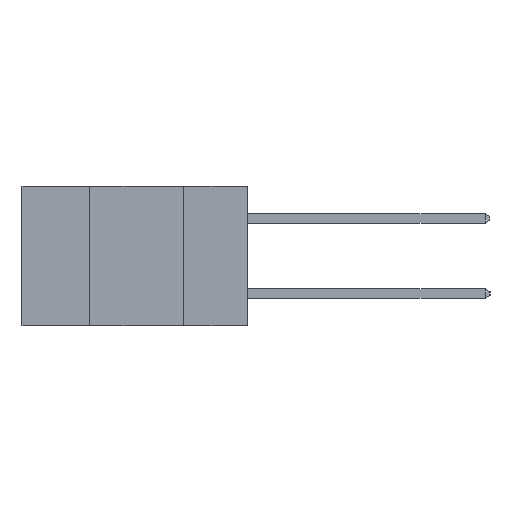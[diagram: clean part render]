
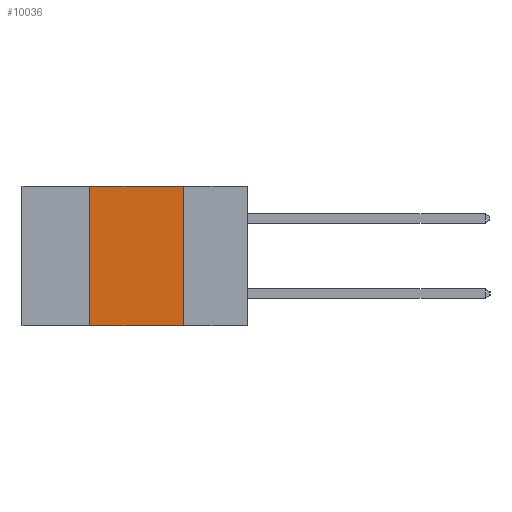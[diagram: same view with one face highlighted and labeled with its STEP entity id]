
A CAD part, left-side view. The second image highlights one B-rep face of the part: STEP entity #10036.
In plain terms, the highlighted planar face has unit normal (-1, 0, 0).
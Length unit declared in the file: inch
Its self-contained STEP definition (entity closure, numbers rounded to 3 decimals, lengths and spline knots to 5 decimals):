
#439 = CARTESIAN_POINT ( 'NONE',  ( 0., 0.42, 0. ) ) ;
#570 = VECTOR ( 'NONE', #14172, 39.37008 ) ;
#571 = DIRECTION ( 'NONE',  ( 0., 0., 1. ) ) ;
#798 = ORIENTED_EDGE ( 'NONE', *, *, #13704, .T. ) ;
#988 = ORIENTED_EDGE ( 'NONE', *, *, #10927, .F. ) ;
#1127 = CARTESIAN_POINT ( 'NONE',  ( 0., 0.6, -0.37 ) ) ;
#1369 = VERTEX_POINT ( 'NONE', #439 ) ;
#2080 = ORIENTED_EDGE ( 'NONE', *, *, #7025, .F. ) ;
#2158 = CARTESIAN_POINT ( 'NONE',  ( 0., 0.42, -0.37 ) ) ;
#2432 = ORIENTED_EDGE ( 'NONE', *, *, #4763, .F. ) ;
#2491 = VERTEX_POINT ( 'NONE', #6785 ) ;
#3468 = DIRECTION ( 'NONE',  ( 0., 0., -1. ) ) ;
#3516 = CARTESIAN_POINT ( 'NONE',  ( 0., 0.17, -0.37 ) ) ;
#4007 = EDGE_LOOP ( 'NONE', ( #2432, #988, #2080, #798 ) ) ;
#4614 = AXIS2_PLACEMENT_3D ( 'NONE', #9665, #9629, #12897 ) ;
#4763 = EDGE_CURVE ( 'NONE', #11511, #11398, #11446, .T. ) ;
#6702 = VECTOR ( 'NONE', #9638, 39.37008 ) ;
#6785 = CARTESIAN_POINT ( 'NONE',  ( 0., 0.42, -0.37 ) ) ;
#7025 = EDGE_CURVE ( 'NONE', #2491, #1369, #11936, .T. ) ;
#7072 = LINE ( 'NONE', #1127, #6702 ) ;
#8431 = VECTOR ( 'NONE', #3468, 39.37008 ) ;
#9294 = VECTOR ( 'NONE', #571, 39.37008 ) ;
#9629 = DIRECTION ( 'NONE',  ( 1., 0., 0. ) ) ;
#9638 = DIRECTION ( 'NONE',  ( 0., -1., 0. ) ) ;
#9665 = CARTESIAN_POINT ( 'NONE',  ( 0., 0.6, 0. ) ) ;
#9682 = PLANE ( 'NONE',  #4614 ) ;
#9752 = LINE ( 'NONE', #14270, #570 ) ;
#10036 = ADVANCED_FACE ( 'NONE', ( #14291 ), #9682, .F. ) ;
#10927 = EDGE_CURVE ( 'NONE', #1369, #11511, #9752, .T. ) ;
#11398 = VERTEX_POINT ( 'NONE', #13919 ) ;
#11446 = LINE ( 'NONE', #3516, #8431 ) ;
#11511 = VERTEX_POINT ( 'NONE', #12046 ) ;
#11936 = LINE ( 'NONE', #2158, #9294 ) ;
#12046 = CARTESIAN_POINT ( 'NONE',  ( 0., 0.17, 0. ) ) ;
#12897 = DIRECTION ( 'NONE',  ( 0., 0., -1. ) ) ;
#13704 = EDGE_CURVE ( 'NONE', #2491, #11398, #7072, .T. ) ;
#13919 = CARTESIAN_POINT ( 'NONE',  ( 0., 0.17, -0.37 ) ) ;
#14172 = DIRECTION ( 'NONE',  ( 0., -1., 0. ) ) ;
#14270 = CARTESIAN_POINT ( 'NONE',  ( 0., 0.6, 0. ) ) ;
#14291 = FACE_OUTER_BOUND ( 'NONE', #4007, .T. ) ;
